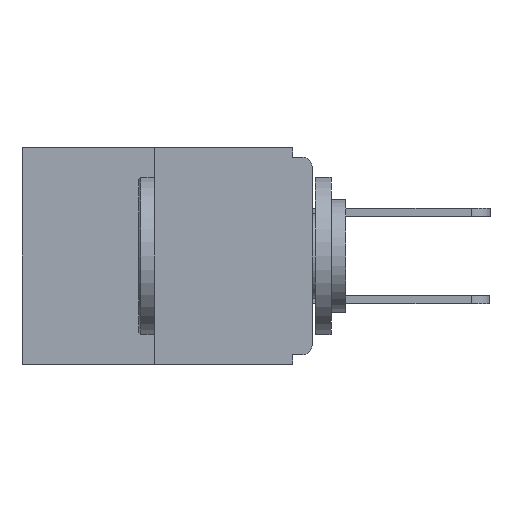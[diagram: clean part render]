
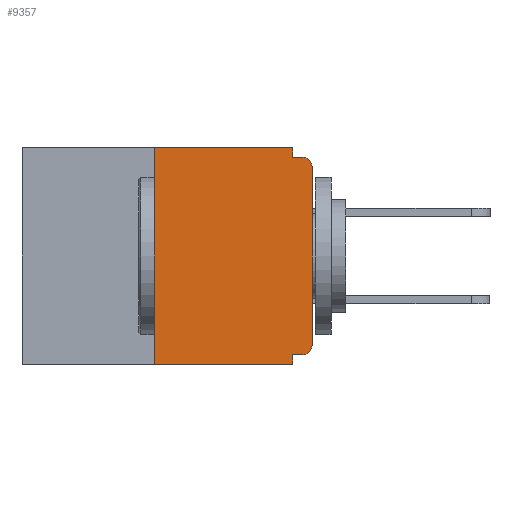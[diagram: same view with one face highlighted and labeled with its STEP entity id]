
A CAD part, left-side view. The second image highlights one B-rep face of the part: STEP entity #9357.
In plain terms, the highlighted planar face has unit normal (-1, 0, 0).
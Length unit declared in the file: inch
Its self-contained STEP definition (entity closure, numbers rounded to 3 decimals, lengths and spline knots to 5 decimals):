
#40 = VERTEX_POINT ( 'NONE', #3684 ) ;
#70 = VECTOR ( 'NONE', #7961, 39.37008 ) ;
#81 = AXIS2_PLACEMENT_3D ( 'NONE', #11425, #8582, #345 ) ;
#203 = PLANE ( 'NONE',  #5772 ) ;
#345 = DIRECTION ( 'NONE',  ( 0., 0., -1. ) ) ;
#415 = CIRCLE ( 'NONE', #81, 0.015 ) ;
#452 = ORIENTED_EDGE ( 'NONE', *, *, #2986, .F. ) ;
#773 = ORIENTED_EDGE ( 'NONE', *, *, #6029, .F. ) ;
#788 = LINE ( 'NONE', #7240, #70 ) ;
#834 = EDGE_CURVE ( 'NONE', #8056, #5337, #415, .T. ) ;
#1176 = FACE_OUTER_BOUND ( 'NONE', #5330, .T. ) ;
#1236 = CARTESIAN_POINT ( 'NONE',  ( 0., 0.031, 0. ) ) ;
#1516 = CARTESIAN_POINT ( 'NONE',  ( 0., 0.015, -0.313 ) ) ;
#1812 = EDGE_CURVE ( 'NONE', #2335, #7235, #4972, .T. ) ;
#2044 = LINE ( 'NONE', #3807, #11900 ) ;
#2160 = DIRECTION ( 'NONE',  ( 0., 0., -1. ) ) ;
#2161 = DIRECTION ( 'NONE',  ( 1., 0., 0. ) ) ;
#2335 = VERTEX_POINT ( 'NONE', #6934 ) ;
#2390 = LINE ( 'NONE', #9901, #7183 ) ;
#2922 = CARTESIAN_POINT ( 'NONE',  ( 0., 0.015, -0.015 ) ) ;
#2944 = EDGE_CURVE ( 'NONE', #11803, #5301, #10639, .T. ) ;
#2986 = EDGE_CURVE ( 'NONE', #11803, #11602, #8884, .T. ) ;
#3061 = ORIENTED_EDGE ( 'NONE', *, *, #3154, .F. ) ;
#3151 = AXIS2_PLACEMENT_3D ( 'NONE', #1516, #11722, #8911 ) ;
#3154 = EDGE_CURVE ( 'NONE', #2335, #5508, #3221, .T. ) ;
#3221 = LINE ( 'NONE', #7394, #9622 ) ;
#3296 = EDGE_CURVE ( 'NONE', #5508, #5301, #11790, .T. ) ;
#3457 = ORIENTED_EDGE ( 'NONE', *, *, #834, .T. ) ;
#3492 = CARTESIAN_POINT ( 'NONE',  ( 0., 0., -0.313 ) ) ;
#3509 = DIRECTION ( 'NONE',  ( 0., -1., 0. ) ) ;
#3534 = CARTESIAN_POINT ( 'NONE',  ( 0., 0.25, 0. ) ) ;
#3684 = CARTESIAN_POINT ( 'NONE',  ( 0., 0.031, 0. ) ) ;
#3807 = CARTESIAN_POINT ( 'NONE',  ( 0., 0., 0. ) ) ;
#4725 = DIRECTION ( 'NONE',  ( 0., 0., 1. ) ) ;
#4972 = CIRCLE ( 'NONE', #3151, 0.015 ) ;
#5134 = CARTESIAN_POINT ( 'NONE',  ( 0., 0.25, -0.343 ) ) ;
#5301 = VERTEX_POINT ( 'NONE', #8570 ) ;
#5330 = EDGE_LOOP ( 'NONE', ( #8970, #452, #6646, #10821, #3061, #6718, #8757, #3457, #773, #5983 ) ) ;
#5337 = VERTEX_POINT ( 'NONE', #2922 ) ;
#5508 = VERTEX_POINT ( 'NONE', #11494 ) ;
#5772 = AXIS2_PLACEMENT_3D ( 'NONE', #6824, #2161, #8591 ) ;
#5819 = VECTOR ( 'NONE', #9375, 39.37008 ) ;
#5983 = ORIENTED_EDGE ( 'NONE', *, *, #8005, .F. ) ;
#6029 = EDGE_CURVE ( 'NONE', #8367, #5337, #2390, .T. ) ;
#6432 = VECTOR ( 'NONE', #9746, 39.37008 ) ;
#6646 = ORIENTED_EDGE ( 'NONE', *, *, #2944, .T. ) ;
#6718 = ORIENTED_EDGE ( 'NONE', *, *, #1812, .T. ) ;
#6824 = CARTESIAN_POINT ( 'NONE',  ( 0., 0.46, 0. ) ) ;
#6934 = CARTESIAN_POINT ( 'NONE',  ( 0., 0.015, -0.328 ) ) ;
#7183 = VECTOR ( 'NONE', #3509, 39.37008 ) ;
#7235 = VERTEX_POINT ( 'NONE', #3492 ) ;
#7240 = CARTESIAN_POINT ( 'NONE',  ( 0., 0.46, 0. ) ) ;
#7394 = CARTESIAN_POINT ( 'NONE',  ( 0., 0., -0.328 ) ) ;
#7577 = CARTESIAN_POINT ( 'NONE',  ( 0., 0.031, -0.343 ) ) ;
#7720 = EDGE_CURVE ( 'NONE', #11602, #40, #788, .T. ) ;
#7961 = DIRECTION ( 'NONE',  ( 0., -1., 0. ) ) ;
#8005 = EDGE_CURVE ( 'NONE', #40, #8367, #9612, .T. ) ;
#8056 = VERTEX_POINT ( 'NONE', #9651 ) ;
#8367 = VERTEX_POINT ( 'NONE', #9761 ) ;
#8570 = CARTESIAN_POINT ( 'NONE',  ( 0., 0.031, -0.343 ) ) ;
#8582 = DIRECTION ( 'NONE',  ( -1., 0., 0. ) ) ;
#8591 = DIRECTION ( 'NONE',  ( 0., 0., -1. ) ) ;
#8757 = ORIENTED_EDGE ( 'NONE', *, *, #9268, .T. ) ;
#8884 = LINE ( 'NONE', #11660, #6432 ) ;
#8911 = DIRECTION ( 'NONE',  ( 0., 0., -1. ) ) ;
#8970 = ORIENTED_EDGE ( 'NONE', *, *, #7720, .F. ) ;
#9268 = EDGE_CURVE ( 'NONE', #7235, #8056, #2044, .T. ) ;
#9317 = VECTOR ( 'NONE', #2160, 39.37008 ) ;
#9357 = ADVANCED_FACE ( 'NONE', ( #1176 ), #203, .F. ) ;
#9375 = DIRECTION ( 'NONE',  ( 0., 0., -1. ) ) ;
#9612 = LINE ( 'NONE', #1236, #9317 ) ;
#9622 = VECTOR ( 'NONE', #10234, 39.37008 ) ;
#9651 = CARTESIAN_POINT ( 'NONE',  ( 0., 0., -0.03 ) ) ;
#9746 = DIRECTION ( 'NONE',  ( 0., 0., 1. ) ) ;
#9761 = CARTESIAN_POINT ( 'NONE',  ( 0., 0.031, -0.015 ) ) ;
#9901 = CARTESIAN_POINT ( 'NONE',  ( 0., 0., -0.015 ) ) ;
#10234 = DIRECTION ( 'NONE',  ( 0., 1., 0. ) ) ;
#10639 = LINE ( 'NONE', #11619, #11937 ) ;
#10641 = DIRECTION ( 'NONE',  ( 0., -1., 0. ) ) ;
#10821 = ORIENTED_EDGE ( 'NONE', *, *, #3296, .F. ) ;
#11425 = CARTESIAN_POINT ( 'NONE',  ( 0., 0.015, -0.03 ) ) ;
#11494 = CARTESIAN_POINT ( 'NONE',  ( 0., 0.031, -0.328 ) ) ;
#11602 = VERTEX_POINT ( 'NONE', #3534 ) ;
#11619 = CARTESIAN_POINT ( 'NONE',  ( 0., 0.46, -0.343 ) ) ;
#11660 = CARTESIAN_POINT ( 'NONE',  ( 0., 0.25, 0. ) ) ;
#11722 = DIRECTION ( 'NONE',  ( -1., 0., 0. ) ) ;
#11790 = LINE ( 'NONE', #7577, #5819 ) ;
#11803 = VERTEX_POINT ( 'NONE', #5134 ) ;
#11900 = VECTOR ( 'NONE', #4725, 39.37008 ) ;
#11937 = VECTOR ( 'NONE', #10641, 39.37008 ) ;
